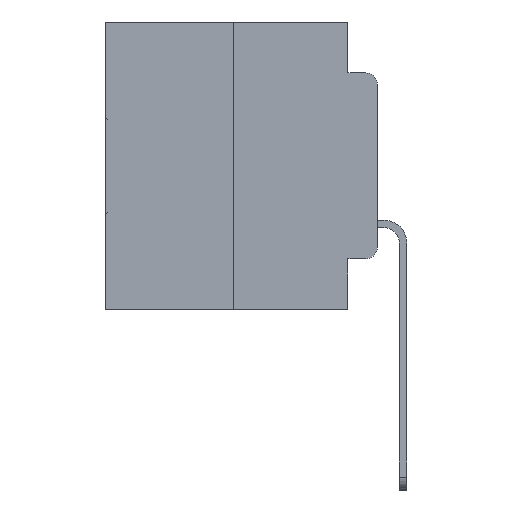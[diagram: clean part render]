
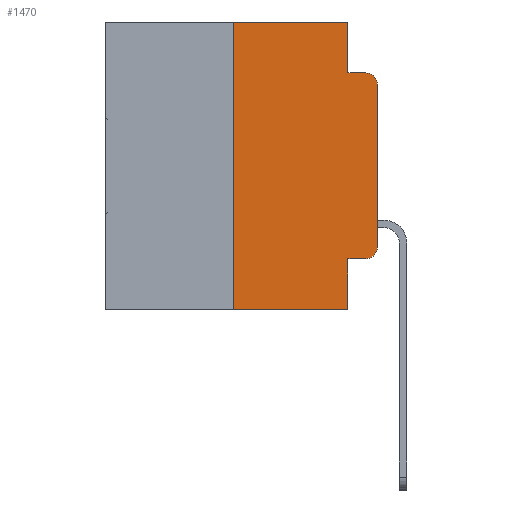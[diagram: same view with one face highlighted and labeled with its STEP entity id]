
A CAD part, left-side view. The second image highlights one B-rep face of the part: STEP entity #1470.
In plain terms, the highlighted planar face has unit normal (-1, 0, 0).
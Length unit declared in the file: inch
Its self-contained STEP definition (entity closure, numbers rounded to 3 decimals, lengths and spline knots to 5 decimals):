
#151 = CARTESIAN_POINT ( 'NONE',  ( 0., 0.051, -0.4115 ) ) ;
#398 = CARTESIAN_POINT ( 'NONE',  ( 0., 0.051, 0. ) ) ;
#570 = VERTEX_POINT ( 'NONE', #24127 ) ;
#989 = LINE ( 'NONE', #28649, #26229 ) ;
#1470 = ADVANCED_FACE ( 'NONE', ( #27361 ), #1614, .F. ) ;
#1586 = VECTOR ( 'NONE', #15758, 39.37008 ) ;
#1614 = PLANE ( 'NONE',  #14745 ) ;
#2095 = EDGE_CURVE ( 'NONE', #10587, #26629, #989, .T. ) ;
#2745 = ORIENTED_EDGE ( 'NONE', *, *, #15010, .F. ) ;
#3160 = CARTESIAN_POINT ( 'NONE',  ( 0., 0.25, 0. ) ) ;
#3861 = CARTESIAN_POINT ( 'NONE',  ( 0., 0.051, 0. ) ) ;
#4188 = LINE ( 'NONE', #23790, #21446 ) ;
#4223 = DIRECTION ( 'NONE',  ( 0., 0., -1. ) ) ;
#4376 = EDGE_CURVE ( 'NONE', #19902, #570, #20881, .T. ) ;
#5404 = CARTESIAN_POINT ( 'NONE',  ( 0., 0.051, -0.0885 ) ) ;
#5435 = EDGE_CURVE ( 'NONE', #26948, #14518, #29029, .T. ) ;
#5764 = ORIENTED_EDGE ( 'NONE', *, *, #23239, .T. ) ;
#6095 = EDGE_CURVE ( 'NONE', #16544, #14518, #4188, .T. ) ;
#6719 = CARTESIAN_POINT ( 'NONE',  ( 0., 0., -0.1085 ) ) ;
#7579 = LINE ( 'NONE', #151, #19231 ) ;
#8684 = DIRECTION ( 'NONE',  ( 0., 0., 1. ) ) ;
#9303 = ORIENTED_EDGE ( 'NONE', *, *, #9737, .T. ) ;
#9555 = CARTESIAN_POINT ( 'NONE',  ( 0., 0.02, -0.1085 ) ) ;
#9737 = EDGE_CURVE ( 'NONE', #570, #15341, #21812, .T. ) ;
#10289 = VECTOR ( 'NONE', #24996, 39.37008 ) ;
#10587 = VERTEX_POINT ( 'NONE', #19288 ) ;
#11128 = VERTEX_POINT ( 'NONE', #25047 ) ;
#11229 = DIRECTION ( 'NONE',  ( 0., 0., -1. ) ) ;
#11901 = DIRECTION ( 'NONE',  ( 0., 0., -1. ) ) ;
#12083 = VERTEX_POINT ( 'NONE', #5404 ) ;
#12556 = CARTESIAN_POINT ( 'NONE',  ( 0., 0.02, -0.3915 ) ) ;
#13473 = EDGE_CURVE ( 'NONE', #16544, #10587, #24453, .T. ) ;
#13526 = CARTESIAN_POINT ( 'NONE',  ( 0., 0.051, 0. ) ) ;
#13725 = CARTESIAN_POINT ( 'NONE',  ( 0., 0.051, -0.4115 ) ) ;
#13811 = CARTESIAN_POINT ( 'NONE',  ( 0., 0.473, 0. ) ) ;
#13833 = EDGE_LOOP ( 'NONE', ( #9303, #29101, #25220, #2745, #14517, #25791, #23265, #15409, #5764, #21815 ) ) ;
#14517 = ORIENTED_EDGE ( 'NONE', *, *, #2095, .F. ) ;
#14518 = VERTEX_POINT ( 'NONE', #29840 ) ;
#14555 = LINE ( 'NONE', #20414, #1586 ) ;
#14745 = AXIS2_PLACEMENT_3D ( 'NONE', #13811, #18400, #4223 ) ;
#14895 = DIRECTION ( 'NONE',  ( 0., 0., -1. ) ) ;
#14962 = DIRECTION ( 'NONE',  ( 0., -1., 0. ) ) ;
#15010 = EDGE_CURVE ( 'NONE', #26629, #12083, #16473, .T. ) ;
#15341 = VERTEX_POINT ( 'NONE', #6719 ) ;
#15409 = ORIENTED_EDGE ( 'NONE', *, *, #5435, .F. ) ;
#15662 = CARTESIAN_POINT ( 'NONE',  ( 0., 0., 0. ) ) ;
#15758 = DIRECTION ( 'NONE',  ( 0., -1., 0. ) ) ;
#15772 = VECTOR ( 'NONE', #8684, 39.37008 ) ;
#16473 = LINE ( 'NONE', #3861, #10289 ) ;
#16544 = VERTEX_POINT ( 'NONE', #28536 ) ;
#17639 = VECTOR ( 'NONE', #24384, 39.37008 ) ;
#18400 = DIRECTION ( 'NONE',  ( 1., 0., 0. ) ) ;
#19157 = DIRECTION ( 'NONE',  ( 0., -1., 0. ) ) ;
#19231 = VECTOR ( 'NONE', #28490, 39.37008 ) ;
#19288 = CARTESIAN_POINT ( 'NONE',  ( 0., 0.25, 0. ) ) ;
#19902 = VERTEX_POINT ( 'NONE', #29694 ) ;
#20414 = CARTESIAN_POINT ( 'NONE',  ( 0., 0.051, -0.0885 ) ) ;
#20881 = CIRCLE ( 'NONE', #23592, 0.02 ) ;
#21446 = VECTOR ( 'NONE', #19157, 39.37008 ) ;
#21812 = LINE ( 'NONE', #15662, #15772 ) ;
#21815 = ORIENTED_EDGE ( 'NONE', *, *, #4376, .T. ) ;
#22987 = VECTOR ( 'NONE', #11229, 39.37008 ) ;
#23239 = EDGE_CURVE ( 'NONE', #26948, #19902, #7579, .T. ) ;
#23265 = ORIENTED_EDGE ( 'NONE', *, *, #6095, .T. ) ;
#23592 = AXIS2_PLACEMENT_3D ( 'NONE', #12556, #28577, #14895 ) ;
#23790 = CARTESIAN_POINT ( 'NONE',  ( 0., 0.473, -0.5 ) ) ;
#24127 = CARTESIAN_POINT ( 'NONE',  ( 0., 0., -0.3915 ) ) ;
#24202 = EDGE_CURVE ( 'NONE', #12083, #11128, #14555, .T. ) ;
#24384 = DIRECTION ( 'NONE',  ( 0., 0., 1. ) ) ;
#24438 = CIRCLE ( 'NONE', #30066, 0.02 ) ;
#24453 = LINE ( 'NONE', #3160, #17639 ) ;
#24996 = DIRECTION ( 'NONE',  ( 0., 0., -1. ) ) ;
#25047 = CARTESIAN_POINT ( 'NONE',  ( 0., 0.02, -0.0885 ) ) ;
#25220 = ORIENTED_EDGE ( 'NONE', *, *, #24202, .F. ) ;
#25671 = DIRECTION ( 'NONE',  ( -1., 0., 0. ) ) ;
#25791 = ORIENTED_EDGE ( 'NONE', *, *, #13473, .F. ) ;
#26229 = VECTOR ( 'NONE', #14962, 39.37008 ) ;
#26629 = VERTEX_POINT ( 'NONE', #398 ) ;
#26948 = VERTEX_POINT ( 'NONE', #13725 ) ;
#27361 = FACE_OUTER_BOUND ( 'NONE', #13833, .T. ) ;
#28490 = DIRECTION ( 'NONE',  ( 0., -1., 0. ) ) ;
#28536 = CARTESIAN_POINT ( 'NONE',  ( 0., 0.25, -0.5 ) ) ;
#28577 = DIRECTION ( 'NONE',  ( -1., 0., 0. ) ) ;
#28649 = CARTESIAN_POINT ( 'NONE',  ( 0., 0.473, 0. ) ) ;
#29029 = LINE ( 'NONE', #13526, #22987 ) ;
#29101 = ORIENTED_EDGE ( 'NONE', *, *, #30241, .T. ) ;
#29694 = CARTESIAN_POINT ( 'NONE',  ( 0., 0.02, -0.4115 ) ) ;
#29840 = CARTESIAN_POINT ( 'NONE',  ( 0., 0.051, -0.5 ) ) ;
#30066 = AXIS2_PLACEMENT_3D ( 'NONE', #9555, #25671, #11901 ) ;
#30241 = EDGE_CURVE ( 'NONE', #15341, #11128, #24438, .T. ) ;
